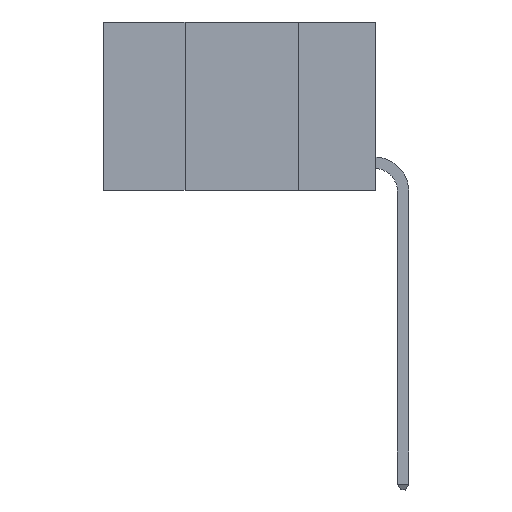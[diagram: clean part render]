
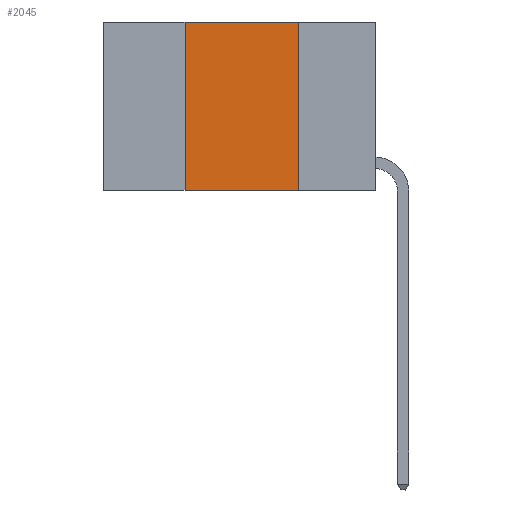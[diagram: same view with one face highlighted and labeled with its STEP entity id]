
A CAD part, left-side view. The second image highlights one B-rep face of the part: STEP entity #2045.
In plain terms, the highlighted planar face has unit normal (-1, 0, 0).
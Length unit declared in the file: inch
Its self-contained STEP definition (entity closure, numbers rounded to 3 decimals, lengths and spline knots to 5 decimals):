
#775 = FACE_OUTER_BOUND ( 'NONE', #23215, .T. ) ;
#1522 = ORIENTED_EDGE ( 'NONE', *, *, #13675, .T. ) ;
#1892 = EDGE_CURVE ( 'NONE', #14686, #21040, #18673, .T. ) ;
#2045 = ADVANCED_FACE ( 'NONE', ( #775 ), #4629, .F. ) ;
#2486 = LINE ( 'NONE', #23100, #14170 ) ;
#4064 = ORIENTED_EDGE ( 'NONE', *, *, #1892, .F. ) ;
#4229 = EDGE_CURVE ( 'NONE', #21040, #11575, #2486, .T. ) ;
#4386 = VECTOR ( 'NONE', #21752, 39.37008 ) ;
#4629 = PLANE ( 'NONE',  #18701 ) ;
#4747 = CARTESIAN_POINT ( 'NONE',  ( 0., 0.6, -0.37 ) ) ;
#5429 = CARTESIAN_POINT ( 'NONE',  ( 0., 0.17, 0. ) ) ;
#5471 = CARTESIAN_POINT ( 'NONE',  ( 0., 0.42, 0. ) ) ;
#6290 = CARTESIAN_POINT ( 'NONE',  ( 0., 0.6, 0. ) ) ;
#7010 = CARTESIAN_POINT ( 'NONE',  ( 0., 0.17, 0. ) ) ;
#8510 = VECTOR ( 'NONE', #12096, 39.37008 ) ;
#11154 = DIRECTION ( 'NONE',  ( 0., 0., 1. ) ) ;
#11383 = LINE ( 'NONE', #4747, #8510 ) ;
#11575 = VERTEX_POINT ( 'NONE', #5429 ) ;
#11634 = DIRECTION ( 'NONE',  ( 1., 0., 0. ) ) ;
#11718 = VECTOR ( 'NONE', #11154, 39.37008 ) ;
#11775 = DIRECTION ( 'NONE',  ( 0., -1., 0. ) ) ;
#11977 = DIRECTION ( 'NONE',  ( 0., 0., -1. ) ) ;
#12096 = DIRECTION ( 'NONE',  ( 0., -1., 0. ) ) ;
#12527 = CARTESIAN_POINT ( 'NONE',  ( 0., 0.42, 0. ) ) ;
#13536 = CARTESIAN_POINT ( 'NONE',  ( 0., 0.42, -0.37 ) ) ;
#13675 = EDGE_CURVE ( 'NONE', #14686, #14550, #11383, .T. ) ;
#14139 = ORIENTED_EDGE ( 'NONE', *, *, #17935, .F. ) ;
#14170 = VECTOR ( 'NONE', #11775, 39.37008 ) ;
#14550 = VERTEX_POINT ( 'NONE', #16114 ) ;
#14686 = VERTEX_POINT ( 'NONE', #13536 ) ;
#16114 = CARTESIAN_POINT ( 'NONE',  ( 0., 0.17, -0.37 ) ) ;
#16227 = LINE ( 'NONE', #7010, #4386 ) ;
#17935 = EDGE_CURVE ( 'NONE', #11575, #14550, #16227, .T. ) ;
#17996 = ORIENTED_EDGE ( 'NONE', *, *, #4229, .F. ) ;
#18673 = LINE ( 'NONE', #5471, #11718 ) ;
#18701 = AXIS2_PLACEMENT_3D ( 'NONE', #6290, #11634, #11977 ) ;
#21040 = VERTEX_POINT ( 'NONE', #12527 ) ;
#21752 = DIRECTION ( 'NONE',  ( 0., 0., -1. ) ) ;
#23100 = CARTESIAN_POINT ( 'NONE',  ( 0., 0.6, 0. ) ) ;
#23215 = EDGE_LOOP ( 'NONE', ( #14139, #17996, #4064, #1522 ) ) ;
